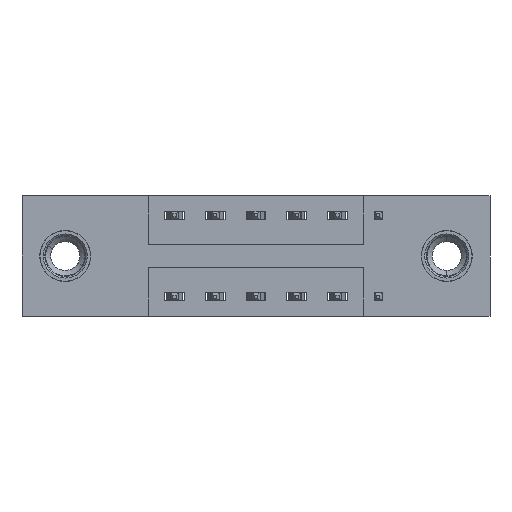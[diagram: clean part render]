
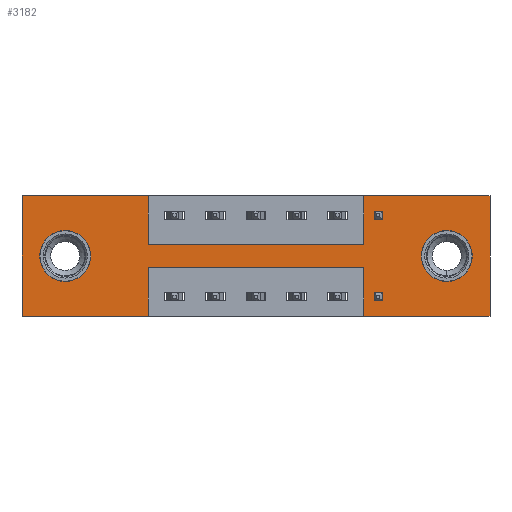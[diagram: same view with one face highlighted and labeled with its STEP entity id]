
A CAD part, front view. The second image highlights one B-rep face of the part: STEP entity #3182.
In plain terms, the highlighted planar face has unit normal (0, -1, 0).
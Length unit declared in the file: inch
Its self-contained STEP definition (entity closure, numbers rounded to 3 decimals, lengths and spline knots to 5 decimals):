
#11 = VERTEX_POINT ( 'NONE', #2830 ) ;
#41 = LINE ( 'NONE', #809, #1223 ) ;
#46 = LINE ( 'NONE', #2998, #7616 ) ;
#112 = EDGE_CURVE ( 'NONE', #4611, #2164, #4220, .T. ) ;
#191 = FACE_BOUND ( 'NONE', #4609, .T. ) ;
#219 = VECTOR ( 'NONE', #3961, 39.37008 ) ;
#229 = DIRECTION ( 'NONE',  ( -1., 0., 0. ) ) ;
#230 = VERTEX_POINT ( 'NONE', #7546 ) ;
#233 = VECTOR ( 'NONE', #609, 39.37008 ) ;
#279 = CARTESIAN_POINT ( 'NONE',  ( 0.3875, 0., -0.37 ) ) ;
#361 = DIRECTION ( 'NONE',  ( 0., 1., 0. ) ) ;
#596 = DIRECTION ( 'NONE',  ( 0., 0., -1. ) ) ;
#609 = DIRECTION ( 'NONE',  ( 0., 0., -1. ) ) ;
#702 = VERTEX_POINT ( 'NONE', #6701 ) ;
#809 = CARTESIAN_POINT ( 'NONE',  ( 0., 0., 0. ) ) ;
#812 = VECTOR ( 'NONE', #3022, 39.37008 ) ;
#844 = CARTESIAN_POINT ( 'NONE',  ( 1.0475, 0., -0.15 ) ) ;
#921 = ORIENTED_EDGE ( 'NONE', *, *, #7374, .F. ) ;
#941 = DIRECTION ( 'NONE',  ( 0., 1., 0. ) ) ;
#948 = DIRECTION ( 'NONE',  ( 0., -1., 0. ) ) ;
#997 = CARTESIAN_POINT ( 'NONE',  ( 0., 0., 0. ) ) ;
#1011 = LINE ( 'NONE', #8848, #812 ) ;
#1029 = EDGE_CURVE ( 'NONE', #1094, #7818, #4345, .T. ) ;
#1089 = ORIENTED_EDGE ( 'NONE', *, *, #1029, .F. ) ;
#1094 = VERTEX_POINT ( 'NONE', #9342 ) ;
#1098 = VERTEX_POINT ( 'NONE', #2248 ) ;
#1223 = VECTOR ( 'NONE', #2993, 39.37008 ) ;
#1228 = VERTEX_POINT ( 'NONE', #8847 ) ;
#1583 = CARTESIAN_POINT ( 'NONE',  ( 1.0475, 0., -0.37 ) ) ;
#1681 = FACE_BOUND ( 'NONE', #8498, .T. ) ;
#1785 = LINE ( 'NONE', #6998, #4762 ) ;
#1808 = VERTEX_POINT ( 'NONE', #5124 ) ;
#1928 = EDGE_CURVE ( 'NONE', #1808, #4046, #3133, .T. ) ;
#2164 = VERTEX_POINT ( 'NONE', #3225 ) ;
#2219 = VECTOR ( 'NONE', #5332, 39.37008 ) ;
#2248 = CARTESIAN_POINT ( 'NONE',  ( 0., 0., -0.37 ) ) ;
#2252 = LINE ( 'NONE', #2979, #9240 ) ;
#2279 = CIRCLE ( 'NONE', #8897, 0.078 ) ;
#2286 = CIRCLE ( 'NONE', #2579, 0.078 ) ;
#2355 = EDGE_CURVE ( 'NONE', #4046, #1094, #6461, .T. ) ;
#2401 = ORIENTED_EDGE ( 'NONE', *, *, #7666, .F. ) ;
#2404 = DIRECTION ( 'NONE',  ( 0., 0., -1. ) ) ;
#2447 = CARTESIAN_POINT ( 'NONE',  ( 0., 0., -0.37 ) ) ;
#2492 = ORIENTED_EDGE ( 'NONE', *, *, #5592, .T. ) ;
#2511 = DIRECTION ( 'NONE',  ( 0., 0., 1. ) ) ;
#2579 = AXIS2_PLACEMENT_3D ( 'NONE', #2892, #4251, #5116 ) ;
#2830 = CARTESIAN_POINT ( 'NONE',  ( 0.1325, 0., -0.107 ) ) ;
#2892 = CARTESIAN_POINT ( 'NONE',  ( 0.1325, 0., -0.185 ) ) ;
#2965 = ORIENTED_EDGE ( 'NONE', *, *, #1928, .F. ) ;
#2979 = CARTESIAN_POINT ( 'NONE',  ( 0.3875, 0., -0.15 ) ) ;
#2993 = DIRECTION ( 'NONE',  ( 0., 0., 1. ) ) ;
#2998 = CARTESIAN_POINT ( 'NONE',  ( 0., 0., -0.37 ) ) ;
#3022 = DIRECTION ( 'NONE',  ( 1., 0., 0. ) ) ;
#3133 = LINE ( 'NONE', #1583, #3304 ) ;
#3182 = ADVANCED_FACE ( 'NONE', ( #1681, #191, #4689 ), #8275, .T. ) ;
#3225 = CARTESIAN_POINT ( 'NONE',  ( 1.3025, 0., -0.107 ) ) ;
#3245 = CARTESIAN_POINT ( 'NONE',  ( 0.1325, 0., -0.185 ) ) ;
#3304 = VECTOR ( 'NONE', #5210, 39.37008 ) ;
#3458 = CARTESIAN_POINT ( 'NONE',  ( 1.0475, 0., -0.22 ) ) ;
#3506 = EDGE_CURVE ( 'NONE', #702, #11, #2286, .T. ) ;
#3604 = LINE ( 'NONE', #4427, #9526 ) ;
#3744 = VERTEX_POINT ( 'NONE', #844 ) ;
#3823 = ORIENTED_EDGE ( 'NONE', *, *, #2355, .F. ) ;
#3954 = ORIENTED_EDGE ( 'NONE', *, *, #6424, .F. ) ;
#3961 = DIRECTION ( 'NONE',  ( 1., 0., 0. ) ) ;
#4046 = VERTEX_POINT ( 'NONE', #3458 ) ;
#4220 = CIRCLE ( 'NONE', #7293, 0.078 ) ;
#4251 = DIRECTION ( 'NONE',  ( 0., 1., 0. ) ) ;
#4345 = LINE ( 'NONE', #7270, #233 ) ;
#4427 = CARTESIAN_POINT ( 'NONE',  ( 1.435, 0., 0. ) ) ;
#4554 = ORIENTED_EDGE ( 'NONE', *, *, #3506, .T. ) ;
#4609 = EDGE_LOOP ( 'NONE', ( #2492, #4554 ) ) ;
#4611 = VERTEX_POINT ( 'NONE', #5355 ) ;
#4689 = FACE_OUTER_BOUND ( 'NONE', #7488, .T. ) ;
#4745 = DIRECTION ( 'NONE',  ( 0., 0., 1. ) ) ;
#4762 = VECTOR ( 'NONE', #4745, 39.37008 ) ;
#4773 = EDGE_CURVE ( 'NONE', #5809, #6334, #9108, .T. ) ;
#4816 = DIRECTION ( 'NONE',  ( 0., 0., -1. ) ) ;
#4841 = ORIENTED_EDGE ( 'NONE', *, *, #8119, .F. ) ;
#4993 = EDGE_CURVE ( 'NONE', #6334, #7856, #9037, .T. ) ;
#5063 = CARTESIAN_POINT ( 'NONE',  ( 1.435, 0., -0.37 ) ) ;
#5116 = DIRECTION ( 'NONE',  ( 0., 0., 1. ) ) ;
#5124 = CARTESIAN_POINT ( 'NONE',  ( 1.0475, 0., -0.37 ) ) ;
#5165 = CARTESIAN_POINT ( 'NONE',  ( 0.3875, 0., 0. ) ) ;
#5210 = DIRECTION ( 'NONE',  ( 0., 0., 1. ) ) ;
#5310 = DIRECTION ( 'NONE',  ( -1., 0., 0. ) ) ;
#5332 = DIRECTION ( 'NONE',  ( 0., 0., -1. ) ) ;
#5355 = CARTESIAN_POINT ( 'NONE',  ( 1.3025, 0., -0.263 ) ) ;
#5383 = ORIENTED_EDGE ( 'NONE', *, *, #6744, .F. ) ;
#5582 = ORIENTED_EDGE ( 'NONE', *, *, #9409, .F. ) ;
#5592 = EDGE_CURVE ( 'NONE', #11, #702, #9159, .T. ) ;
#5738 = CARTESIAN_POINT ( 'NONE',  ( 0.3875, 0., -0.22 ) ) ;
#5809 = VERTEX_POINT ( 'NONE', #8282 ) ;
#5889 = EDGE_CURVE ( 'NONE', #7818, #1098, #46, .T. ) ;
#6195 = DIRECTION ( 'NONE',  ( 0., 1., 0. ) ) ;
#6334 = VERTEX_POINT ( 'NONE', #5165 ) ;
#6424 = EDGE_CURVE ( 'NONE', #7954, #1808, #6843, .T. ) ;
#6461 = LINE ( 'NONE', #5738, #8004 ) ;
#6701 = CARTESIAN_POINT ( 'NONE',  ( 0.1325, 0., -0.263 ) ) ;
#6728 = ORIENTED_EDGE ( 'NONE', *, *, #4993, .F. ) ;
#6744 = EDGE_CURVE ( 'NONE', #1228, #230, #1011, .T. ) ;
#6843 = LINE ( 'NONE', #2447, #7295 ) ;
#6998 = CARTESIAN_POINT ( 'NONE',  ( 1.0475, 0., 0. ) ) ;
#7270 = CARTESIAN_POINT ( 'NONE',  ( 0.3875, 0., -0.37 ) ) ;
#7293 = AXIS2_PLACEMENT_3D ( 'NONE', #9097, #941, #7697 ) ;
#7295 = VECTOR ( 'NONE', #229, 39.37008 ) ;
#7374 = EDGE_CURVE ( 'NONE', #3744, #1228, #1785, .T. ) ;
#7488 = EDGE_LOOP ( 'NONE', ( #1089, #3823, #2965, #3954, #5582, #5383, #921, #4841, #6728, #7530, #2401, #8257 ) ) ;
#7530 = ORIENTED_EDGE ( 'NONE', *, *, #4773, .F. ) ;
#7546 = CARTESIAN_POINT ( 'NONE',  ( 1.435, 0., 0. ) ) ;
#7616 = VECTOR ( 'NONE', #5310, 39.37008 ) ;
#7665 = ORIENTED_EDGE ( 'NONE', *, *, #9269, .T. ) ;
#7666 = EDGE_CURVE ( 'NONE', #1098, #5809, #41, .T. ) ;
#7697 = DIRECTION ( 'NONE',  ( 0., 0., -1. ) ) ;
#7778 = CARTESIAN_POINT ( 'NONE',  ( 1.3025, 0., -0.185 ) ) ;
#7794 = CARTESIAN_POINT ( 'NONE',  ( 0.3875, 0., -0.15 ) ) ;
#7818 = VERTEX_POINT ( 'NONE', #279 ) ;
#7856 = VERTEX_POINT ( 'NONE', #7794 ) ;
#7954 = VERTEX_POINT ( 'NONE', #5063 ) ;
#8004 = VECTOR ( 'NONE', #8654, 39.37008 ) ;
#8119 = EDGE_CURVE ( 'NONE', #7856, #3744, #2252, .T. ) ;
#8203 = ORIENTED_EDGE ( 'NONE', *, *, #112, .T. ) ;
#8220 = DIRECTION ( 'NONE',  ( 1., 0., 0. ) ) ;
#8257 = ORIENTED_EDGE ( 'NONE', *, *, #5889, .F. ) ;
#8275 = PLANE ( 'NONE',  #8884 ) ;
#8282 = CARTESIAN_POINT ( 'NONE',  ( 0., 0., 0. ) ) ;
#8498 = EDGE_LOOP ( 'NONE', ( #7665, #8203 ) ) ;
#8654 = DIRECTION ( 'NONE',  ( -1., 0., 0. ) ) ;
#8847 = CARTESIAN_POINT ( 'NONE',  ( 1.0475, 0., 0. ) ) ;
#8848 = CARTESIAN_POINT ( 'NONE',  ( 0., 0., 0. ) ) ;
#8884 = AXIS2_PLACEMENT_3D ( 'NONE', #9511, #948, #2404 ) ;
#8897 = AXIS2_PLACEMENT_3D ( 'NONE', #7778, #361, #4816 ) ;
#9037 = LINE ( 'NONE', #9083, #2219 ) ;
#9083 = CARTESIAN_POINT ( 'NONE',  ( 0.3875, 0., 0. ) ) ;
#9097 = CARTESIAN_POINT ( 'NONE',  ( 1.3025, 0., -0.185 ) ) ;
#9108 = LINE ( 'NONE', #997, #219 ) ;
#9159 = CIRCLE ( 'NONE', #9323, 0.078 ) ;
#9240 = VECTOR ( 'NONE', #8220, 39.37008 ) ;
#9269 = EDGE_CURVE ( 'NONE', #2164, #4611, #2279, .T. ) ;
#9323 = AXIS2_PLACEMENT_3D ( 'NONE', #3245, #6195, #2511 ) ;
#9342 = CARTESIAN_POINT ( 'NONE',  ( 0.3875, 0., -0.22 ) ) ;
#9409 = EDGE_CURVE ( 'NONE', #230, #7954, #3604, .T. ) ;
#9511 = CARTESIAN_POINT ( 'NONE',  ( 0., 0., -0.37 ) ) ;
#9526 = VECTOR ( 'NONE', #596, 39.37008 ) ;
